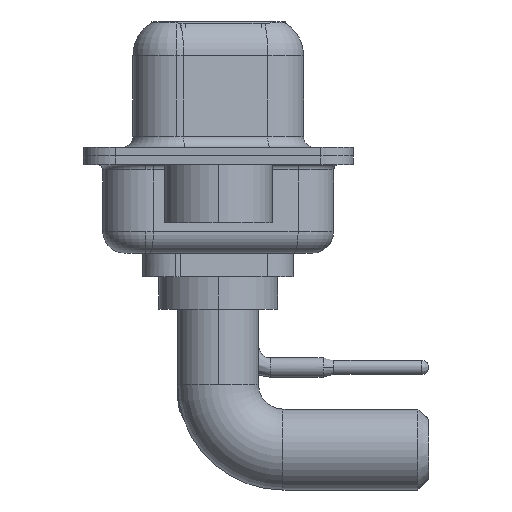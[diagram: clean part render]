
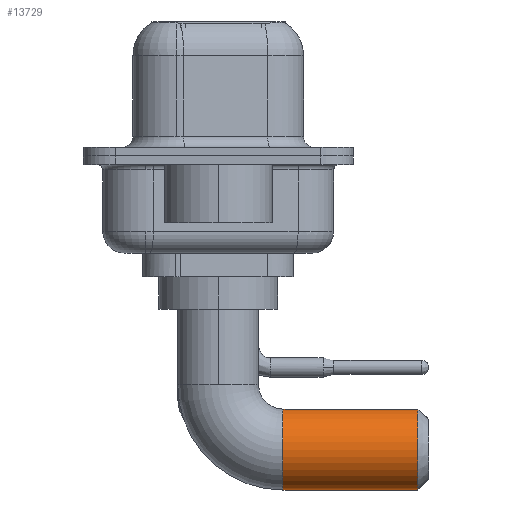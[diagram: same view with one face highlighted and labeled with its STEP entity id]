
A CAD part, left-side view. The second image highlights one B-rep face of the part: STEP entity #13729.
In plain terms, the highlighted cylindrical face has radius 1.875 mm (diameter 3.75 mm), a partial arc.
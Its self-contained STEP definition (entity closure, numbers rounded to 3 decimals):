
#1416 = VERTEX_POINT ( 'NONE', #23320 ) ;
#3413 = FACE_OUTER_BOUND ( 'NONE', #20420, .T. ) ;
#3759 = AXIS2_PLACEMENT_3D ( 'NONE', #21562, #15998, #21321 ) ;
#4124 = VERTEX_POINT ( 'NONE', #18905 ) ;
#5010 = EDGE_CURVE ( 'NONE', #11290, #17072, #13139, .T. ) ;
#5318 = LINE ( 'NONE', #8559, #17747 ) ;
#5948 = DIRECTION ( 'NONE',  ( 0., -1., 0. ) ) ;
#6170 = ORIENTED_EDGE ( 'NONE', *, *, #10350, .T. ) ;
#7496 = DIRECTION ( 'NONE',  ( 0., -1., 0. ) ) ;
#7538 = ORIENTED_EDGE ( 'NONE', *, *, #14064, .T. ) ;
#7699 = AXIS2_PLACEMENT_3D ( 'NONE', #22018, #11020, #23579 ) ;
#8080 = CIRCLE ( 'NONE', #7699, 1.875 ) ;
#8559 = CARTESIAN_POINT ( 'NONE',  ( 0., -3., -8.375 ) ) ;
#10350 = EDGE_CURVE ( 'NONE', #1416, #4124, #5318, .T. ) ;
#11020 = DIRECTION ( 'NONE',  ( 0., 1., 0. ) ) ;
#11290 = VERTEX_POINT ( 'NONE', #19576 ) ;
#11420 = CARTESIAN_POINT ( 'NONE',  ( 0., -9.25, -4.625 ) ) ;
#13066 = ORIENTED_EDGE ( 'NONE', *, *, #15928, .T. ) ;
#13139 = LINE ( 'NONE', #20519, #19119 ) ;
#13729 = ADVANCED_FACE ( 'NONE', ( #3413 ), #20146, .T. ) ;
#13765 = AXIS2_PLACEMENT_3D ( 'NONE', #14585, #7496, #22184 ) ;
#14064 = EDGE_CURVE ( 'NONE', #11290, #1416, #15654, .T. ) ;
#14585 = CARTESIAN_POINT ( 'NONE',  ( 0., -3., -6.5 ) ) ;
#15654 = CIRCLE ( 'NONE', #3759, 1.875 ) ;
#15928 = EDGE_CURVE ( 'NONE', #4124, #17072, #8080, .T. ) ;
#15998 = DIRECTION ( 'NONE',  ( 0., -1., 0. ) ) ;
#16372 = DIRECTION ( 'NONE',  ( 0., -1., 0. ) ) ;
#17072 = VERTEX_POINT ( 'NONE', #11420 ) ;
#17747 = VECTOR ( 'NONE', #16372, 1000. ) ;
#18905 = CARTESIAN_POINT ( 'NONE',  ( 0., -9.25, -8.375 ) ) ;
#19119 = VECTOR ( 'NONE', #5948, 1000. ) ;
#19576 = CARTESIAN_POINT ( 'NONE',  ( 0., -3., -4.625 ) ) ;
#20146 = CYLINDRICAL_SURFACE ( 'NONE', #13765, 1.875 ) ;
#20280 = ORIENTED_EDGE ( 'NONE', *, *, #5010, .F. ) ;
#20420 = EDGE_LOOP ( 'NONE', ( #20280, #7538, #6170, #13066 ) ) ;
#20519 = CARTESIAN_POINT ( 'NONE',  ( 0., -3., -4.625 ) ) ;
#21321 = DIRECTION ( 'NONE',  ( -1., 0., 0. ) ) ;
#21562 = CARTESIAN_POINT ( 'NONE',  ( 0., -3., -6.5 ) ) ;
#22018 = CARTESIAN_POINT ( 'NONE',  ( 0., -9.25, -6.5 ) ) ;
#22184 = DIRECTION ( 'NONE',  ( 0., 0., -1. ) ) ;
#23320 = CARTESIAN_POINT ( 'NONE',  ( 0., -3., -8.375 ) ) ;
#23579 = DIRECTION ( 'NONE',  ( 0., 0., -1. ) ) ;
